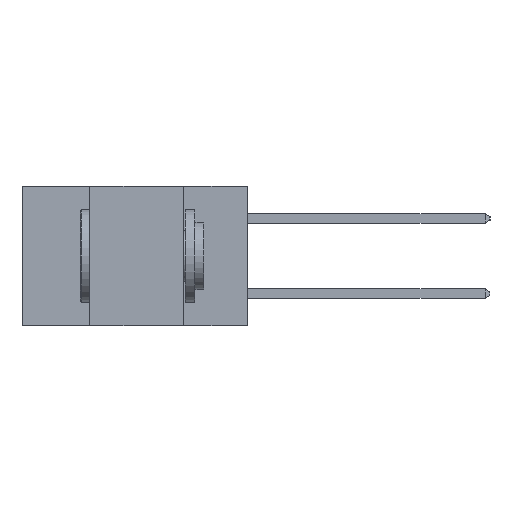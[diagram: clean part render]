
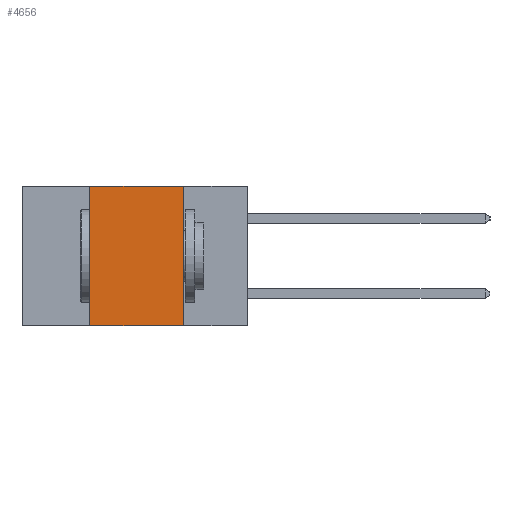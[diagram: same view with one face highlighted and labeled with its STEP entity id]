
A CAD part, left-side view. The second image highlights one B-rep face of the part: STEP entity #4656.
In plain terms, the highlighted planar face has unit normal (-1, 0, 0).
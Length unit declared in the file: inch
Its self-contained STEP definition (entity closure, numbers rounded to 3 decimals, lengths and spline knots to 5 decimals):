
#1249 = EDGE_CURVE ( 'NONE', #6976, #9963, #25524, .T. ) ;
#1306 = ORIENTED_EDGE ( 'NONE', *, *, #2649, .F. ) ;
#2649 = EDGE_CURVE ( 'NONE', #9963, #14062, #8632, .T. ) ;
#2725 = CARTESIAN_POINT ( 'NONE',  ( 0., 0.42, -0.37 ) ) ;
#4656 = ADVANCED_FACE ( 'NONE', ( #9900 ), #20471, .F. ) ;
#5492 = EDGE_CURVE ( 'NONE', #14062, #21594, #9808, .T. ) ;
#6260 = ORIENTED_EDGE ( 'NONE', *, *, #5492, .F. ) ;
#6262 = DIRECTION ( 'NONE',  ( 0., 0., -1. ) ) ;
#6545 = DIRECTION ( 'NONE',  ( 0., 0., 1. ) ) ;
#6959 = ORIENTED_EDGE ( 'NONE', *, *, #1249, .F. ) ;
#6976 = VERTEX_POINT ( 'NONE', #27217 ) ;
#6998 = CARTESIAN_POINT ( 'NONE',  ( 0., 0.6, -0.37 ) ) ;
#7723 = CARTESIAN_POINT ( 'NONE',  ( 0., 0.6, 0. ) ) ;
#7808 = DIRECTION ( 'NONE',  ( 1., 0., 0. ) ) ;
#7978 = VECTOR ( 'NONE', #26005, 39.37008 ) ;
#8632 = LINE ( 'NONE', #26047, #7978 ) ;
#8685 = CARTESIAN_POINT ( 'NONE',  ( 0., 0.17, -0.37 ) ) ;
#9134 = DIRECTION ( 'NONE',  ( 0., -1., 0. ) ) ;
#9291 = EDGE_LOOP ( 'NONE', ( #6260, #1306, #6959, #23805 ) ) ;
#9808 = LINE ( 'NONE', #26925, #25288 ) ;
#9900 = FACE_OUTER_BOUND ( 'NONE', #9291, .T. ) ;
#9963 = VERTEX_POINT ( 'NONE', #22827 ) ;
#14062 = VERTEX_POINT ( 'NONE', #17996 ) ;
#14890 = LINE ( 'NONE', #6998, #25379 ) ;
#17996 = CARTESIAN_POINT ( 'NONE',  ( 0., 0.17, 0. ) ) ;
#19318 = VECTOR ( 'NONE', #6545, 39.37008 ) ;
#20471 = PLANE ( 'NONE',  #25939 ) ;
#21594 = VERTEX_POINT ( 'NONE', #8685 ) ;
#22564 = DIRECTION ( 'NONE',  ( 0., 0., -1. ) ) ;
#22827 = CARTESIAN_POINT ( 'NONE',  ( 0., 0.42, 0. ) ) ;
#23805 = ORIENTED_EDGE ( 'NONE', *, *, #27234, .T. ) ;
#25288 = VECTOR ( 'NONE', #6262, 39.37008 ) ;
#25379 = VECTOR ( 'NONE', #9134, 39.37008 ) ;
#25524 = LINE ( 'NONE', #2725, #19318 ) ;
#25939 = AXIS2_PLACEMENT_3D ( 'NONE', #7723, #7808, #22564 ) ;
#26005 = DIRECTION ( 'NONE',  ( 0., -1., 0. ) ) ;
#26047 = CARTESIAN_POINT ( 'NONE',  ( 0., 0.6, 0. ) ) ;
#26925 = CARTESIAN_POINT ( 'NONE',  ( 0., 0.17, -0.37 ) ) ;
#27217 = CARTESIAN_POINT ( 'NONE',  ( 0., 0.42, -0.37 ) ) ;
#27234 = EDGE_CURVE ( 'NONE', #6976, #21594, #14890, .T. ) ;
